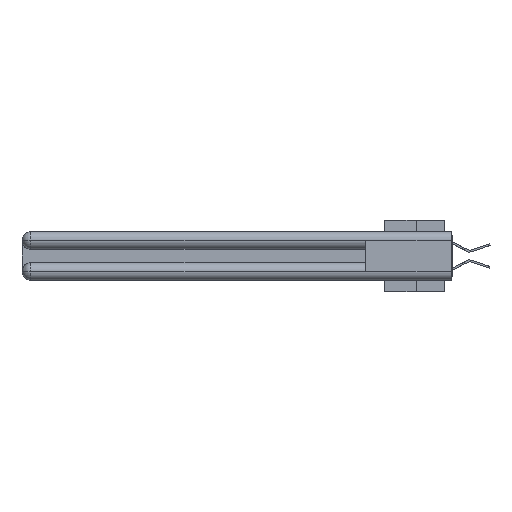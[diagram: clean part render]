
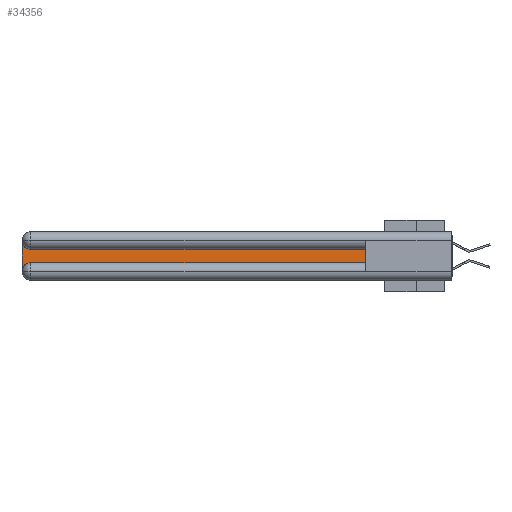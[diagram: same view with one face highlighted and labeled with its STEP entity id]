
A CAD part, left-side view. The second image highlights one B-rep face of the part: STEP entity #34356.
In plain terms, the highlighted planar face has unit normal (-1, 0, 0).
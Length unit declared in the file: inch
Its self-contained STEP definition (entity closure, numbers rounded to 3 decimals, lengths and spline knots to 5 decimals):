
#330 = CARTESIAN_POINT ( 'NONE',  ( 0.075, 0.6, -0.1225 ) ) ;
#1273 = CARTESIAN_POINT ( 'NONE',  ( 0.075, 3., -0.1225 ) ) ;
#1354 = LINE ( 'NONE', #3646, #14539 ) ;
#1676 = VECTOR ( 'NONE', #2013, 39.37008 ) ;
#2013 = DIRECTION ( 'NONE',  ( 0., -1., 0. ) ) ;
#2630 = LINE ( 'NONE', #30226, #1676 ) ;
#2717 = ORIENTED_EDGE ( 'NONE', *, *, #10961, .T. ) ;
#2958 = DIRECTION ( 'NONE',  ( 0., 0., -1. ) ) ;
#3556 = VERTEX_POINT ( 'NONE', #16120 ) ;
#3646 = CARTESIAN_POINT ( 'NONE',  ( 0.075, 3., -0.2175 ) ) ;
#3787 = CARTESIAN_POINT ( 'NONE',  ( 0.075, 2.94, -0.1225 ) ) ;
#4404 = PLANE ( 'NONE',  #22218 ) ;
#6014 = DIRECTION ( 'NONE',  ( 1., 0., 0. ) ) ;
#6165 = VERTEX_POINT ( 'NONE', #22824 ) ;
#7995 = VERTEX_POINT ( 'NONE', #32103 ) ;
#8700 = CARTESIAN_POINT ( 'NONE',  ( 0.075, 0.6, -0.2175 ) ) ;
#10961 = EDGE_CURVE ( 'NONE', #3556, #7995, #30107, .T. ) ;
#11424 = VECTOR ( 'NONE', #28549, 39.37008 ) ;
#12170 = CARTESIAN_POINT ( 'NONE',  ( 0.075, 2.94, -0.0625 ) ) ;
#12668 = ORIENTED_EDGE ( 'NONE', *, *, #38549, .T. ) ;
#12685 = ORIENTED_EDGE ( 'NONE', *, *, #34688, .T. ) ;
#13013 = VERTEX_POINT ( 'NONE', #3787 ) ;
#13695 = DIRECTION ( 'NONE',  ( 1., 0., 0. ) ) ;
#14539 = VECTOR ( 'NONE', #16212, 39.37008 ) ;
#16120 = CARTESIAN_POINT ( 'NONE',  ( 0.075, 3., -0.2775 ) ) ;
#16212 = DIRECTION ( 'NONE',  ( 0., 0., -1. ) ) ;
#16766 = AXIS2_PLACEMENT_3D ( 'NONE', #27925, #30787, #2958 ) ;
#18094 = VERTEX_POINT ( 'NONE', #8700 ) ;
#18810 = FACE_OUTER_BOUND ( 'NONE', #32812, .T. ) ;
#19450 = EDGE_CURVE ( 'NONE', #7995, #18094, #2630, .T. ) ;
#21345 = DIRECTION ( 'NONE',  ( 0., 0., -1. ) ) ;
#22218 = AXIS2_PLACEMENT_3D ( 'NONE', #1273, #13695, #26876 ) ;
#22824 = CARTESIAN_POINT ( 'NONE',  ( 0.075, 3., -0.0625 ) ) ;
#23317 = VERTEX_POINT ( 'NONE', #37677 ) ;
#24896 = AXIS2_PLACEMENT_3D ( 'NONE', #12170, #6014, #21345 ) ;
#26876 = DIRECTION ( 'NONE',  ( 0., 0., -1. ) ) ;
#27249 = CIRCLE ( 'NONE', #24896, 0.06 ) ;
#27639 = CARTESIAN_POINT ( 'NONE',  ( 0.075, 0.6, -0.2175 ) ) ;
#27925 = CARTESIAN_POINT ( 'NONE',  ( 0.075, 2.94, -0.2775 ) ) ;
#28465 = ORIENTED_EDGE ( 'NONE', *, *, #29379, .T. ) ;
#28549 = DIRECTION ( 'NONE',  ( 0., 1., 0. ) ) ;
#29379 = EDGE_CURVE ( 'NONE', #6165, #3556, #1354, .T. ) ;
#30081 = LINE ( 'NONE', #330, #11424 ) ;
#30107 = CIRCLE ( 'NONE', #16766, 0.06 ) ;
#30226 = CARTESIAN_POINT ( 'NONE',  ( 0.075, 0.6, -0.2175 ) ) ;
#30787 = DIRECTION ( 'NONE',  ( 1., 0., 0. ) ) ;
#31568 = EDGE_CURVE ( 'NONE', #23317, #13013, #30081, .T. ) ;
#31825 = ORIENTED_EDGE ( 'NONE', *, *, #19450, .T. ) ;
#32103 = CARTESIAN_POINT ( 'NONE',  ( 0.075, 2.94, -0.2175 ) ) ;
#32803 = LINE ( 'NONE', #27639, #39127 ) ;
#32812 = EDGE_LOOP ( 'NONE', ( #37727, #12685, #28465, #2717, #31825, #12668 ) ) ;
#34356 = ADVANCED_FACE ( 'NONE', ( #18810 ), #4404, .F. ) ;
#34688 = EDGE_CURVE ( 'NONE', #13013, #6165, #27249, .T. ) ;
#37608 = DIRECTION ( 'NONE',  ( 0., 0., 1. ) ) ;
#37677 = CARTESIAN_POINT ( 'NONE',  ( 0.075, 0.6, -0.1225 ) ) ;
#37727 = ORIENTED_EDGE ( 'NONE', *, *, #31568, .T. ) ;
#38549 = EDGE_CURVE ( 'NONE', #18094, #23317, #32803, .T. ) ;
#39127 = VECTOR ( 'NONE', #37608, 39.37008 ) ;
